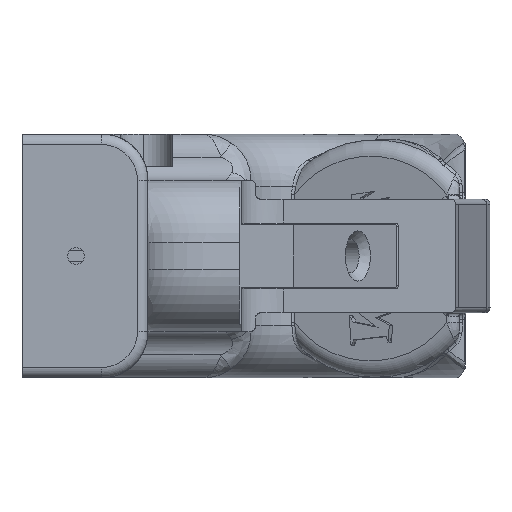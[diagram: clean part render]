
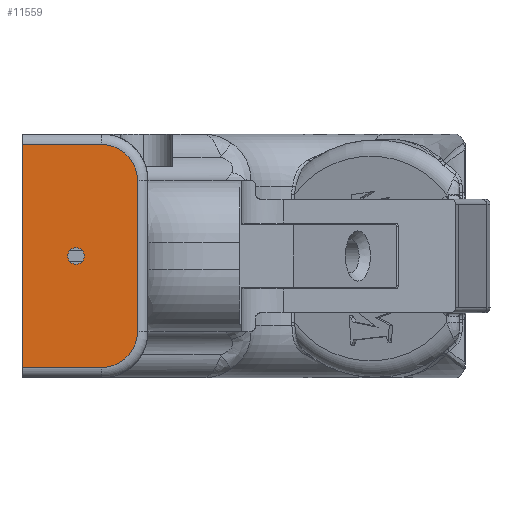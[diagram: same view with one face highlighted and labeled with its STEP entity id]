
A CAD part, left-side view. The second image highlights one B-rep face of the part: STEP entity #11559.
In plain terms, the highlighted planar face has unit normal (-1, 0, 0).
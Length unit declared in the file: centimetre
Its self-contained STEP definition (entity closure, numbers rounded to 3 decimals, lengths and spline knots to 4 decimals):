
#534=CIRCLE($,#12215,0.125);
#537=CIRCLE($,#12220,0.547);
#541=CIRCLE($,#12232,0.547);
#669=FACE_BOUND($,#2514,.T.);
#1814=FACE_OUTER_BOUND($,#2513,.T.);
#2513=EDGE_LOOP($,(#10329,#10330,#10331,#10332,#10333,#10334));
#2514=EDGE_LOOP($,(#10335));
#3339=LINE($,#28323,#4276);
#3444=LINE($,#29392,#4381);
#3445=LINE($,#29394,#4382);
#3446=LINE($,#29395,#4383);
#4276=VECTOR($,#14412,2.3019);
#4381=VECTOR($,#14843,1.212);
#4382=VECTOR($,#14844,3.3958);
#4383=VECTOR($,#14845,1.212);
#5368=VERTEX_POINT($,#28317);
#5369=VERTEX_POINT($,#28320);
#5370=VERTEX_POINT($,#28322);
#5371=VERTEX_POINT($,#28326);
#5381=VERTEX_POINT($,#28353);
#5492=VERTEX_POINT($,#29391);
#5493=VERTEX_POINT($,#29393);
#6933=EDGE_CURVE($,#5368,#5368,#534,.T.);
#6935=EDGE_CURVE($,#5369,#5370,#3339,.T.);
#6937=EDGE_CURVE($,#5370,#5371,#537,.T.);
#6951=EDGE_CURVE($,#5381,#5369,#541,.T.);
#7146=EDGE_CURVE($,#5492,#5381,#3444,.T.);
#7147=EDGE_CURVE($,#5492,#5493,#3445,.T.);
#7148=EDGE_CURVE($,#5371,#5493,#3446,.T.);
#10329=ORIENTED_EDGE($,*,*,#7146,.F.);
#10330=ORIENTED_EDGE($,*,*,#7147,.T.);
#10331=ORIENTED_EDGE($,*,*,#7148,.F.);
#10332=ORIENTED_EDGE($,*,*,#6937,.F.);
#10333=ORIENTED_EDGE($,*,*,#6935,.F.);
#10334=ORIENTED_EDGE($,*,*,#6951,.F.);
#10335=ORIENTED_EDGE($,*,*,#6933,.T.);
#10950=PLANE($,#12380);
#11559=ADVANCED_FACE($,(#1814,#669),#10950,.T.);
#12215=AXIS2_PLACEMENT_3D($,#28318,#14406,#14407);
#12220=AXIS2_PLACEMENT_3D($,#28327,#14417,#14418);
#12232=AXIS2_PLACEMENT_3D($,#28355,#14447,#14448);
#12380=AXIS2_PLACEMENT_3D($,#29390,#14841,#14842);
#14406=DIRECTION('center_axis',(1.,0.,0.));
#14407=DIRECTION('ref_axis',(0.,0.,
-1.));
#14412=DIRECTION($,(0.,0.,-1.));
#14417=DIRECTION('center_axis',(1.,0.,0.));
#14418=DIRECTION('ref_axis',(0.,-0.707,
-0.707));
#14447=DIRECTION('center_axis',(1.,0.,0.));
#14448=DIRECTION('ref_axis',(0.,-0.707,0.707));
#14841=DIRECTION('center_axis',(-1.,0.,0.));
#14842=DIRECTION('ref_axis',(0.,0.,1.));
#14843=DIRECTION($,(0.,-1.,0.));
#14844=DIRECTION($,(0.,0.,-1.));
#14845=DIRECTION($,(0.,1.,0.));
#28317=CARTESIAN_POINT('',(-19.1173,-0.2633,0.125));
#28318=CARTESIAN_POINT('Origin',(-19.1173,-0.2633,0.));
#28320=CARTESIAN_POINT('',(-19.1173,-1.2004,1.1509));
#28322=CARTESIAN_POINT('',(-19.1173,-1.2004,-1.1509));
#28323=CARTESIAN_POINT($,(-19.1173,-1.2004,-1.1509));
#28326=CARTESIAN_POINT('',(-19.1173,-0.6534,-1.6979));
#28327=CARTESIAN_POINT('Origin',(-19.1173,-0.6534,-1.1509));
#28353=CARTESIAN_POINT('',(-19.1173,-0.6534,1.6979));
#28355=CARTESIAN_POINT('Origin',(-19.1173,-0.6534,1.1509));
#29390=CARTESIAN_POINT('Origin',(-19.1173,-0.0777,
-1.1509));
#29391=CARTESIAN_POINT('',(-19.1173,0.5586,1.6979));
#29392=CARTESIAN_POINT($,(-19.1173,0.2405,1.6979));
#29393=CARTESIAN_POINT('',(-19.1173,0.5586,-1.6979));
#29394=CARTESIAN_POINT($,(-19.1173,0.5586,-1.7583));
#29395=CARTESIAN_POINT($,(-19.1173,0.2405,-1.6979));
